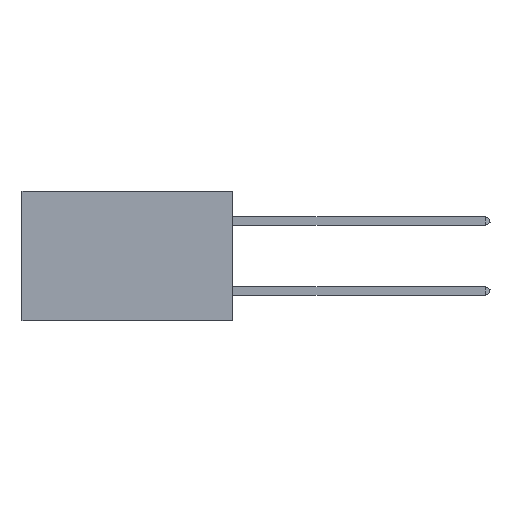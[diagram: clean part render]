
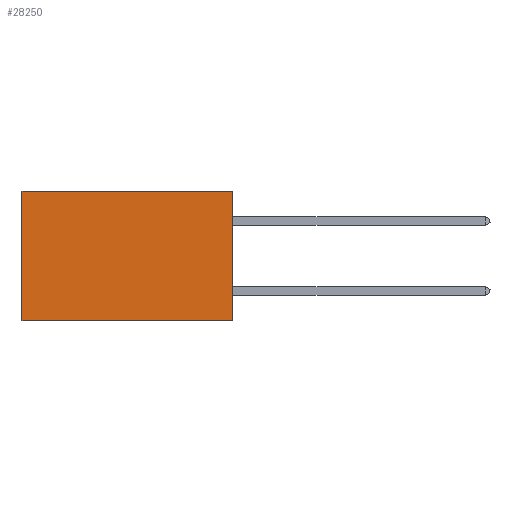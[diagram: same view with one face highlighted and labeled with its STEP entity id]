
A CAD part, left-side view. The second image highlights one B-rep face of the part: STEP entity #28250.
In plain terms, the highlighted planar face has unit normal (-1, 0, 0).
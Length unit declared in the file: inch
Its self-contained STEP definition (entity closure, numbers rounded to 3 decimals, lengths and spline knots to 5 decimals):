
#23 = CARTESIAN_POINT ( 'NONE',  ( 0.2875, 0., -0.37 ) ) ;
#77 = VECTOR ( 'NONE', #29516, 39.37008 ) ;
#805 = LINE ( 'NONE', #15723, #77 ) ;
#2909 = CARTESIAN_POINT ( 'NONE',  ( 0.2875, 0., 0. ) ) ;
#4707 = EDGE_CURVE ( 'NONE', #25002, #10635, #29625, .T. ) ;
#5754 = CARTESIAN_POINT ( 'NONE',  ( 0.2875, 0., 0. ) ) ;
#6324 = LINE ( 'NONE', #26418, #12669 ) ;
#6633 = LINE ( 'NONE', #9251, #29560 ) ;
#8780 = DIRECTION ( 'NONE',  ( 1., 0., 0. ) ) ;
#8825 = EDGE_CURVE ( 'NONE', #25002, #24112, #805, .T. ) ;
#9251 = CARTESIAN_POINT ( 'NONE',  ( 0.2875, 0., -0.37 ) ) ;
#9468 = ORIENTED_EDGE ( 'NONE', *, *, #22841, .F. ) ;
#10635 = VERTEX_POINT ( 'NONE', #22253 ) ;
#11094 = CARTESIAN_POINT ( 'NONE',  ( 0.2875, 0., 0. ) ) ;
#11989 = VECTOR ( 'NONE', #21780, 39.37008 ) ;
#12411 = ORIENTED_EDGE ( 'NONE', *, *, #4707, .T. ) ;
#12533 = DIRECTION ( 'NONE',  ( 0., 0., -1. ) ) ;
#12669 = VECTOR ( 'NONE', #12533, 39.37008 ) ;
#13479 = CARTESIAN_POINT ( 'NONE',  ( 0.2875, 0.6, -0.37 ) ) ;
#14309 = VERTEX_POINT ( 'NONE', #13479 ) ;
#15292 = AXIS2_PLACEMENT_3D ( 'NONE', #11094, #8780, #25124 ) ;
#15723 = CARTESIAN_POINT ( 'NONE',  ( 0.2875, 0., 0. ) ) ;
#17419 = ORIENTED_EDGE ( 'NONE', *, *, #21695, .T. ) ;
#19651 = ORIENTED_EDGE ( 'NONE', *, *, #8825, .F. ) ;
#20883 = FACE_OUTER_BOUND ( 'NONE', #29319, .T. ) ;
#21695 = EDGE_CURVE ( 'NONE', #10635, #14309, #6324, .T. ) ;
#21780 = DIRECTION ( 'NONE',  ( 0., 1., 0. ) ) ;
#22253 = CARTESIAN_POINT ( 'NONE',  ( 0.2875, 0.6, 0. ) ) ;
#22841 = EDGE_CURVE ( 'NONE', #24112, #14309, #6633, .T. ) ;
#22863 = PLANE ( 'NONE',  #15292 ) ;
#23416 = DIRECTION ( 'NONE',  ( 0., 1., 0. ) ) ;
#24112 = VERTEX_POINT ( 'NONE', #23 ) ;
#25002 = VERTEX_POINT ( 'NONE', #5754 ) ;
#25124 = DIRECTION ( 'NONE',  ( 0., 0., -1. ) ) ;
#26418 = CARTESIAN_POINT ( 'NONE',  ( 0.2875, 0.6, 0. ) ) ;
#28250 = ADVANCED_FACE ( 'NONE', ( #20883 ), #22863, .F. ) ;
#29319 = EDGE_LOOP ( 'NONE', ( #17419, #9468, #19651, #12411 ) ) ;
#29516 = DIRECTION ( 'NONE',  ( 0., 0., -1. ) ) ;
#29560 = VECTOR ( 'NONE', #23416, 39.37008 ) ;
#29625 = LINE ( 'NONE', #2909, #11989 ) ;
